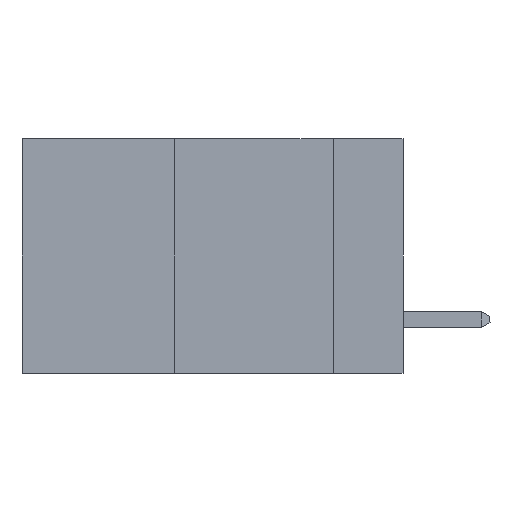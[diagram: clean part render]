
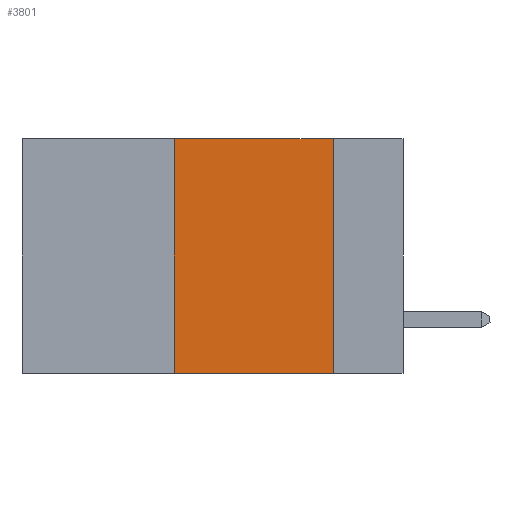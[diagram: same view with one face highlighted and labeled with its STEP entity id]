
A CAD part, left-side view. The second image highlights one B-rep face of the part: STEP entity #3801.
In plain terms, the highlighted planar face has unit normal (-1, 0, 0).
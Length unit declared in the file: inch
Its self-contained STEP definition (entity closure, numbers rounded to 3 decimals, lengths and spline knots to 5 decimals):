
#264 = VERTEX_POINT ( 'NONE', #4998 ) ;
#2112 = EDGE_CURVE ( 'NONE', #4754, #2910, #11041, .T. ) ;
#2179 = ORIENTED_EDGE ( 'NONE', *, *, #6820, .F. ) ;
#2910 = VERTEX_POINT ( 'NONE', #11527 ) ;
#2988 = CARTESIAN_POINT ( 'NONE',  ( 0., 0.6, 0. ) ) ;
#3257 = DIRECTION ( 'NONE',  ( 0., 0., 1. ) ) ;
#3268 = ORIENTED_EDGE ( 'NONE', *, *, #2112, .T. ) ;
#3714 = PLANE ( 'NONE',  #10706 ) ;
#3801 = ADVANCED_FACE ( 'NONE', ( #7860 ), #3714, .F. ) ;
#3918 = DIRECTION ( 'NONE',  ( 0., 0., -1. ) ) ;
#4481 = CARTESIAN_POINT ( 'NONE',  ( 0., 0.6, 0. ) ) ;
#4754 = VERTEX_POINT ( 'NONE', #7592 ) ;
#4922 = EDGE_LOOP ( 'NONE', ( #2179, #12723, #5371, #3268 ) ) ;
#4998 = CARTESIAN_POINT ( 'NONE',  ( 0., 0.36, 0. ) ) ;
#5371 = ORIENTED_EDGE ( 'NONE', *, *, #7041, .F. ) ;
#5475 = VECTOR ( 'NONE', #7144, 39.37008 ) ;
#5619 = LINE ( 'NONE', #11088, #12991 ) ;
#6396 = VECTOR ( 'NONE', #8096, 39.37008 ) ;
#6594 = DIRECTION ( 'NONE',  ( 1., 0., 0. ) ) ;
#6820 = EDGE_CURVE ( 'NONE', #9805, #2910, #8094, .T. ) ;
#7041 = EDGE_CURVE ( 'NONE', #4754, #264, #5619, .T. ) ;
#7144 = DIRECTION ( 'NONE',  ( 0., 0., -1. ) ) ;
#7592 = CARTESIAN_POINT ( 'NONE',  ( 0., 0.36, -0.37 ) ) ;
#7860 = FACE_OUTER_BOUND ( 'NONE', #4922, .T. ) ;
#8094 = LINE ( 'NONE', #11866, #5475 ) ;
#8096 = DIRECTION ( 'NONE',  ( 0., -1., 0. ) ) ;
#8563 = CARTESIAN_POINT ( 'NONE',  ( 0., 0.11, 0. ) ) ;
#9805 = VERTEX_POINT ( 'NONE', #8563 ) ;
#10230 = EDGE_CURVE ( 'NONE', #264, #9805, #12034, .T. ) ;
#10706 = AXIS2_PLACEMENT_3D ( 'NONE', #4481, #6594, #3918 ) ;
#11041 = LINE ( 'NONE', #12527, #13230 ) ;
#11088 = CARTESIAN_POINT ( 'NONE',  ( 0., 0.36, 0. ) ) ;
#11527 = CARTESIAN_POINT ( 'NONE',  ( 0., 0.11, -0.37 ) ) ;
#11866 = CARTESIAN_POINT ( 'NONE',  ( 0., 0.11, 0. ) ) ;
#12034 = LINE ( 'NONE', #2988, #6396 ) ;
#12527 = CARTESIAN_POINT ( 'NONE',  ( 0., 0.6, -0.37 ) ) ;
#12723 = ORIENTED_EDGE ( 'NONE', *, *, #10230, .F. ) ;
#12771 = DIRECTION ( 'NONE',  ( 0., -1., 0. ) ) ;
#12991 = VECTOR ( 'NONE', #3257, 39.37008 ) ;
#13230 = VECTOR ( 'NONE', #12771, 39.37008 ) ;
